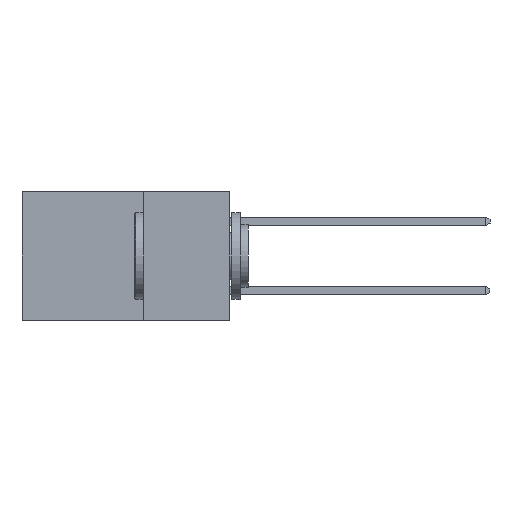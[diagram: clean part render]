
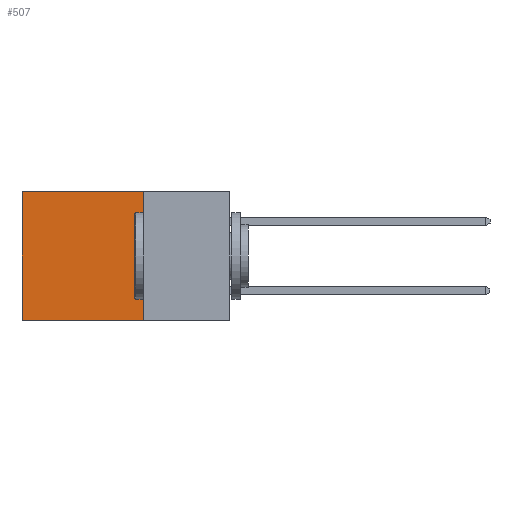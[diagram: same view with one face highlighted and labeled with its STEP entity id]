
A CAD part, left-side view. The second image highlights one B-rep face of the part: STEP entity #507.
In plain terms, the highlighted planar face has unit normal (-1, 0, 0).
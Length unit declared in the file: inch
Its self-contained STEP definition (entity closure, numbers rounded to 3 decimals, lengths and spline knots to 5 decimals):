
#317 = PLANE ( 'NONE',  #1737 ) ;
#395 = DIRECTION ( 'NONE',  ( 0., 0., -1. ) ) ;
#507 = ADVANCED_FACE ( 'NONE', ( #8867 ), #317, .F. ) ;
#1505 = CARTESIAN_POINT ( 'NONE',  ( 0.298, 0.25, 0. ) ) ;
#1686 = DIRECTION ( 'NONE',  ( 1., 0., 0. ) ) ;
#1737 = AXIS2_PLACEMENT_3D ( 'NONE', #1505, #1686, #10005 ) ;
#1835 = VERTEX_POINT ( 'NONE', #6252 ) ;
#2384 = EDGE_CURVE ( 'NONE', #14152, #5301, #12980, .T. ) ;
#3015 = ORIENTED_EDGE ( 'NONE', *, *, #9934, .T. ) ;
#3183 = VERTEX_POINT ( 'NONE', #5607 ) ;
#3356 = ORIENTED_EDGE ( 'NONE', *, *, #2384, .F. ) ;
#4416 = LINE ( 'NONE', #7323, #12749 ) ;
#4891 = EDGE_CURVE ( 'NONE', #1835, #14152, #5148, .T. ) ;
#5148 = LINE ( 'NONE', #9679, #10462 ) ;
#5165 = VECTOR ( 'NONE', #6370, 39.37008 ) ;
#5301 = VERTEX_POINT ( 'NONE', #11884 ) ;
#5607 = CARTESIAN_POINT ( 'NONE',  ( 0.298, 0.6, 0. ) ) ;
#6252 = CARTESIAN_POINT ( 'NONE',  ( 0.298, 0.25, 0. ) ) ;
#6370 = DIRECTION ( 'NONE',  ( 0., 1., 0. ) ) ;
#6374 = CARTESIAN_POINT ( 'NONE',  ( 0.298, 0.25, 0. ) ) ;
#6544 = CARTESIAN_POINT ( 'NONE',  ( 0.298, 0.25, -0.37 ) ) ;
#7236 = VECTOR ( 'NONE', #12555, 39.37008 ) ;
#7323 = CARTESIAN_POINT ( 'NONE',  ( 0.298, 0.6, 0. ) ) ;
#7362 = ORIENTED_EDGE ( 'NONE', *, *, #4891, .F. ) ;
#7636 = DIRECTION ( 'NONE',  ( 0., 0., -1. ) ) ;
#8867 = FACE_OUTER_BOUND ( 'NONE', #11247, .T. ) ;
#9679 = CARTESIAN_POINT ( 'NONE',  ( 0.298, 0.25, 0. ) ) ;
#9934 = EDGE_CURVE ( 'NONE', #1835, #3183, #10823, .T. ) ;
#10005 = DIRECTION ( 'NONE',  ( 0., 0., -1. ) ) ;
#10462 = VECTOR ( 'NONE', #7636, 39.37008 ) ;
#10823 = LINE ( 'NONE', #6374, #5165 ) ;
#11247 = EDGE_LOOP ( 'NONE', ( #14130, #3356, #7362, #3015 ) ) ;
#11884 = CARTESIAN_POINT ( 'NONE',  ( 0.298, 0.6, -0.37 ) ) ;
#12481 = EDGE_CURVE ( 'NONE', #3183, #5301, #4416, .T. ) ;
#12555 = DIRECTION ( 'NONE',  ( 0., 1., 0. ) ) ;
#12679 = CARTESIAN_POINT ( 'NONE',  ( 0.298, 0.25, -0.37 ) ) ;
#12749 = VECTOR ( 'NONE', #395, 39.37008 ) ;
#12980 = LINE ( 'NONE', #12679, #7236 ) ;
#14130 = ORIENTED_EDGE ( 'NONE', *, *, #12481, .T. ) ;
#14152 = VERTEX_POINT ( 'NONE', #6544 ) ;
